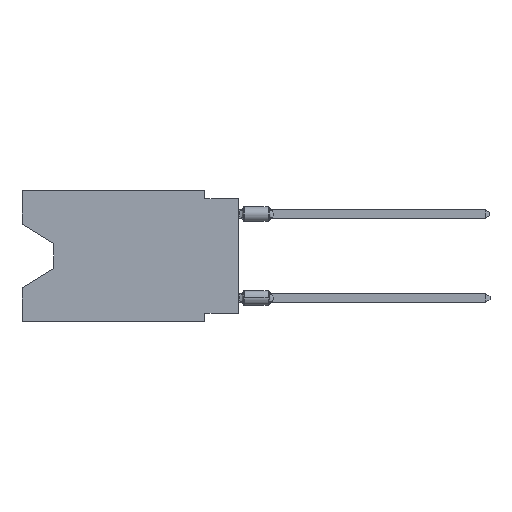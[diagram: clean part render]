
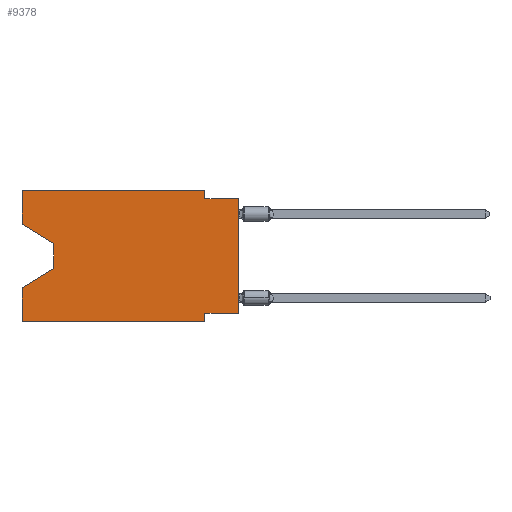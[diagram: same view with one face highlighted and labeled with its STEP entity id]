
A CAD part, left-side view. The second image highlights one B-rep face of the part: STEP entity #9378.
In plain terms, the highlighted planar face has unit normal (-1, 0, 0).
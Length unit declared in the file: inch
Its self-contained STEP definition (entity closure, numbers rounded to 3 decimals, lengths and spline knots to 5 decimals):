
#334 = EDGE_CURVE ( 'NONE', #4817, #32138, #26880, .T. ) ;
#562 = PLANE ( 'NONE',  #21332 ) ;
#832 = CARTESIAN_POINT ( 'NONE',  ( 0., 0.645, -0.39 ) ) ;
#1223 = LINE ( 'NONE', #29818, #1924 ) ;
#1638 = EDGE_CURVE ( 'NONE', #22595, #7246, #29653, .T. ) ;
#1924 = VECTOR ( 'NONE', #24124, 39.37008 ) ;
#2079 = ORIENTED_EDGE ( 'NONE', *, *, #33147, .F. ) ;
#2610 = DIRECTION ( 'NONE',  ( 0., -1., 0. ) ) ;
#3305 = CARTESIAN_POINT ( 'NONE',  ( 0., 0.1, 0. ) ) ;
#3410 = VERTEX_POINT ( 'NONE', #20338 ) ;
#3992 = EDGE_CURVE ( 'NONE', #27176, #27449, #26479, .T. ) ;
#3999 = LINE ( 'NONE', #30345, #11989 ) ;
#4611 = DIRECTION ( 'NONE',  ( 0., 0., -1. ) ) ;
#4817 = VERTEX_POINT ( 'NONE', #32354 ) ;
#5310 = LINE ( 'NONE', #30982, #10191 ) ;
#6100 = DIRECTION ( 'NONE',  ( 0., -1., 0. ) ) ;
#6248 = ORIENTED_EDGE ( 'NONE', *, *, #24128, .F. ) ;
#6454 = VECTOR ( 'NONE', #4611, 39.37008 ) ;
#6583 = LINE ( 'NONE', #9341, #12572 ) ;
#6687 = CARTESIAN_POINT ( 'NONE',  ( 0., 0.645, -0.28975 ) ) ;
#6741 = DIRECTION ( 'NONE',  ( 0., 0., 1. ) ) ;
#7246 = VERTEX_POINT ( 'NONE', #6687 ) ;
#7386 = ORIENTED_EDGE ( 'NONE', *, *, #18610, .T. ) ;
#8666 = LINE ( 'NONE', #26756, #24729 ) ;
#8852 = VECTOR ( 'NONE', #2610, 39.37008 ) ;
#9341 = CARTESIAN_POINT ( 'NONE',  ( 0., 0., -0.025 ) ) ;
#9378 = ADVANCED_FACE ( 'NONE', ( #13310 ), #562, .F. ) ;
#9413 = LINE ( 'NONE', #30423, #19873 ) ;
#9503 = EDGE_CURVE ( 'NONE', #30462, #4817, #3999, .T. ) ;
#9518 = DIRECTION ( 'NONE',  ( 0., -1., 0. ) ) ;
#10191 = VECTOR ( 'NONE', #15820, 39.37008 ) ;
#10972 = DIRECTION ( 'NONE',  ( 0., 0., 1. ) ) ;
#11989 = VECTOR ( 'NONE', #6741, 39.37008 ) ;
#12150 = VECTOR ( 'NONE', #29318, 39.37008 ) ;
#12572 = VECTOR ( 'NONE', #9518, 39.37008 ) ;
#12764 = CARTESIAN_POINT ( 'NONE',  ( 0., 0.55, -0.232 ) ) ;
#12925 = LINE ( 'NONE', #15176, #16580 ) ;
#13310 = FACE_OUTER_BOUND ( 'NONE', #25370, .T. ) ;
#13615 = ORIENTED_EDGE ( 'NONE', *, *, #28473, .F. ) ;
#13646 = DIRECTION ( 'NONE',  ( 1., 0., 0. ) ) ;
#13755 = CARTESIAN_POINT ( 'NONE',  ( 0., 0.1, -0.365 ) ) ;
#13950 = DIRECTION ( 'NONE',  ( 0., 0., 1. ) ) ;
#14456 = ORIENTED_EDGE ( 'NONE', *, *, #334, .F. ) ;
#14684 = EDGE_CURVE ( 'NONE', #17875, #7246, #16363, .T. ) ;
#14891 = ORIENTED_EDGE ( 'NONE', *, *, #20396, .T. ) ;
#15176 = CARTESIAN_POINT ( 'NONE',  ( 0., 0., -0.365 ) ) ;
#15820 = DIRECTION ( 'NONE',  ( 0., 0., -1. ) ) ;
#16256 = LINE ( 'NONE', #26418, #6454 ) ;
#16363 = LINE ( 'NONE', #24796, #28659 ) ;
#16414 = VERTEX_POINT ( 'NONE', #20099 ) ;
#16508 = CARTESIAN_POINT ( 'NONE',  ( 0., 0., -0.025 ) ) ;
#16580 = VECTOR ( 'NONE', #28788, 39.37008 ) ;
#17346 = DIRECTION ( 'NONE',  ( 0., 0., -1. ) ) ;
#17754 = VECTOR ( 'NONE', #10972, 39.37008 ) ;
#17875 = VERTEX_POINT ( 'NONE', #832 ) ;
#17957 = VERTEX_POINT ( 'NONE', #13755 ) ;
#18406 = VERTEX_POINT ( 'NONE', #32005 ) ;
#18610 = EDGE_CURVE ( 'NONE', #3410, #22595, #16256, .T. ) ;
#18647 = CARTESIAN_POINT ( 'NONE',  ( 0., 0.645, 0. ) ) ;
#19147 = CARTESIAN_POINT ( 'NONE',  ( 0., 0.645, 0. ) ) ;
#19873 = VECTOR ( 'NONE', #17346, 39.37008 ) ;
#20099 = CARTESIAN_POINT ( 'NONE',  ( 0., 0.1, -0.025 ) ) ;
#20338 = CARTESIAN_POINT ( 'NONE',  ( 0., 0.55, -0.158 ) ) ;
#20396 = EDGE_CURVE ( 'NONE', #17875, #18406, #8666, .T. ) ;
#21332 = AXIS2_PLACEMENT_3D ( 'NONE', #18647, #13646, #31552 ) ;
#21653 = CARTESIAN_POINT ( 'NONE',  ( 0., 0., 0. ) ) ;
#22520 = EDGE_CURVE ( 'NONE', #27176, #17957, #12925, .T. ) ;
#22595 = VERTEX_POINT ( 'NONE', #12764 ) ;
#23892 = EDGE_CURVE ( 'NONE', #30462, #3410, #1223, .T. ) ;
#24124 = DIRECTION ( 'NONE',  ( 0., -0.855, -0.519 ) ) ;
#24128 = EDGE_CURVE ( 'NONE', #17957, #18406, #5310, .T. ) ;
#24138 = CARTESIAN_POINT ( 'NONE',  ( 0., 0.55, -0.232 ) ) ;
#24729 = VECTOR ( 'NONE', #6100, 39.37008 ) ;
#24796 = CARTESIAN_POINT ( 'NONE',  ( 0., 0.645, 0. ) ) ;
#25370 = EDGE_LOOP ( 'NONE', ( #26166, #7386, #28047, #32485, #14891, #6248, #31625, #26023, #13615, #2079, #14456, #31285 ) ) ;
#26023 = ORIENTED_EDGE ( 'NONE', *, *, #3992, .T. ) ;
#26166 = ORIENTED_EDGE ( 'NONE', *, *, #23892, .T. ) ;
#26418 = CARTESIAN_POINT ( 'NONE',  ( 0., 0.55, -0.158 ) ) ;
#26479 = LINE ( 'NONE', #21653, #17754 ) ;
#26756 = CARTESIAN_POINT ( 'NONE',  ( 0., 0.645, -0.39 ) ) ;
#26880 = LINE ( 'NONE', #19147, #8852 ) ;
#27176 = VERTEX_POINT ( 'NONE', #27727 ) ;
#27449 = VERTEX_POINT ( 'NONE', #16508 ) ;
#27727 = CARTESIAN_POINT ( 'NONE',  ( 0., 0., -0.365 ) ) ;
#28047 = ORIENTED_EDGE ( 'NONE', *, *, #1638, .T. ) ;
#28473 = EDGE_CURVE ( 'NONE', #16414, #27449, #6583, .T. ) ;
#28659 = VECTOR ( 'NONE', #13950, 39.37008 ) ;
#28788 = DIRECTION ( 'NONE',  ( 0., 1., 0. ) ) ;
#29318 = DIRECTION ( 'NONE',  ( 0., 0.855, -0.519 ) ) ;
#29653 = LINE ( 'NONE', #24138, #12150 ) ;
#29818 = CARTESIAN_POINT ( 'NONE',  ( 0., 0.645, -0.10025 ) ) ;
#30345 = CARTESIAN_POINT ( 'NONE',  ( 0., 0.645, 0. ) ) ;
#30423 = CARTESIAN_POINT ( 'NONE',  ( 0., 0.1, 0. ) ) ;
#30462 = VERTEX_POINT ( 'NONE', #32093 ) ;
#30982 = CARTESIAN_POINT ( 'NONE',  ( 0., 0.1, -0.39 ) ) ;
#31285 = ORIENTED_EDGE ( 'NONE', *, *, #9503, .F. ) ;
#31552 = DIRECTION ( 'NONE',  ( 0., 0., -1. ) ) ;
#31625 = ORIENTED_EDGE ( 'NONE', *, *, #22520, .F. ) ;
#32005 = CARTESIAN_POINT ( 'NONE',  ( 0., 0.1, -0.39 ) ) ;
#32093 = CARTESIAN_POINT ( 'NONE',  ( 0., 0.645, -0.10025 ) ) ;
#32138 = VERTEX_POINT ( 'NONE', #3305 ) ;
#32354 = CARTESIAN_POINT ( 'NONE',  ( 0., 0.645, 0. ) ) ;
#32485 = ORIENTED_EDGE ( 'NONE', *, *, #14684, .F. ) ;
#33147 = EDGE_CURVE ( 'NONE', #32138, #16414, #9413, .T. ) ;
